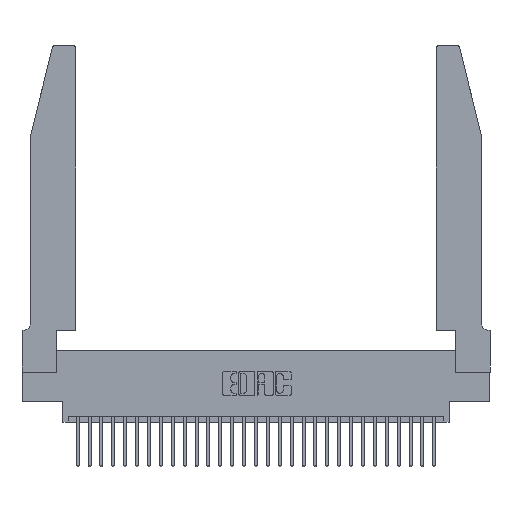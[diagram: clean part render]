
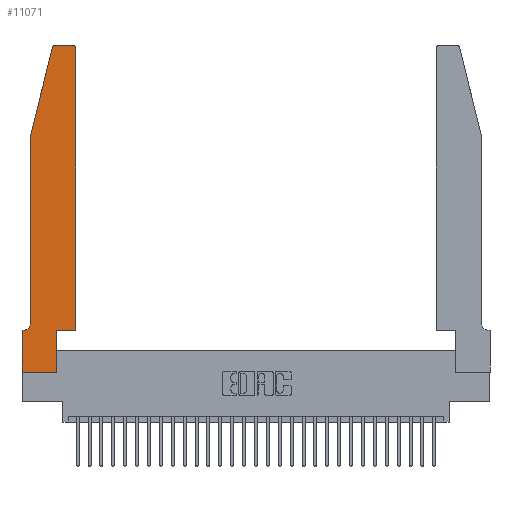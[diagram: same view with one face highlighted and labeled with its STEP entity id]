
A CAD part, top view. The second image highlights one B-rep face of the part: STEP entity #11071.
In plain terms, the highlighted planar face has unit normal (0, 0, 1).
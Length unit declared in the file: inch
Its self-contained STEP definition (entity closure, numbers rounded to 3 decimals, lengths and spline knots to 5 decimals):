
#51 = VECTOR ( 'NONE', #8601, 39.37008 ) ;
#865 = CARTESIAN_POINT ( 'NONE',  ( 0.0755, 2., 0.37 ) ) ;
#918 = LINE ( 'NONE', #25785, #24794 ) ;
#925 = LINE ( 'NONE', #14193, #5953 ) ;
#1254 = VERTEX_POINT ( 'NONE', #4482 ) ;
#1478 = ORIENTED_EDGE ( 'NONE', *, *, #30125, .T. ) ;
#1538 = DIRECTION ( 'NONE',  ( -1., 0., 0. ) ) ;
#1739 = CARTESIAN_POINT ( 'NONE',  ( 0.25487, 2.72718, 0.37 ) ) ;
#1925 = CARTESIAN_POINT ( 'NONE',  ( 0.0755, 0.42, 0.37 ) ) ;
#2300 = DIRECTION ( 'NONE',  ( 1., 0., 0. ) ) ;
#2882 = EDGE_CURVE ( 'NONE', #4517, #6202, #20335, .T. ) ;
#3135 = DIRECTION ( 'NONE',  ( -0.239, -0.971, 0. ) ) ;
#4482 = CARTESIAN_POINT ( 'NONE',  ( 0.0055, 0.35, 0.37 ) ) ;
#4517 = VERTEX_POINT ( 'NONE', #14096 ) ;
#4570 = DIRECTION ( 'NONE',  ( 0., 1., 0. ) ) ;
#5003 = LINE ( 'NONE', #26126, #16939 ) ;
#5183 = VECTOR ( 'NONE', #3135, 39.37008 ) ;
#5503 = VECTOR ( 'NONE', #7867, 39.37008 ) ;
#5849 = CARTESIAN_POINT ( 'NONE',  ( 0.2865, 0.35, 0.37 ) ) ;
#5953 = VECTOR ( 'NONE', #23533, 39.37008 ) ;
#6163 = ORIENTED_EDGE ( 'NONE', *, *, #2882, .T. ) ;
#6202 = VERTEX_POINT ( 'NONE', #11108 ) ;
#6253 = PLANE ( 'NONE',  #24596 ) ;
#6389 = EDGE_CURVE ( 'NONE', #26405, #24461, #918, .T. ) ;
#6524 = AXIS2_PLACEMENT_3D ( 'NONE', #22715, #8539, #25035 ) ;
#6534 = ORIENTED_EDGE ( 'NONE', *, *, #22010, .T. ) ;
#6748 = VECTOR ( 'NONE', #19270, 39.37008 ) ;
#7050 = VERTEX_POINT ( 'NONE', #28063 ) ;
#7363 = CIRCLE ( 'NONE', #26044, 0.07 ) ;
#7867 = DIRECTION ( 'NONE',  ( 0., -1., 0. ) ) ;
#8454 = CARTESIAN_POINT ( 'NONE',  ( 0., 0.35, 0.37 ) ) ;
#8539 = DIRECTION ( 'NONE',  ( 0., 0., 1. ) ) ;
#8601 = DIRECTION ( 'NONE',  ( -1., 0., 0. ) ) ;
#8653 = CARTESIAN_POINT ( 'NONE',  ( 0., 0.35, 0.37 ) ) ;
#8923 = ORIENTED_EDGE ( 'NONE', *, *, #17089, .T. ) ;
#9465 = CARTESIAN_POINT ( 'NONE',  ( 0.2865, 0., 0.37 ) ) ;
#10026 = LINE ( 'NONE', #17082, #21863 ) ;
#10037 = ORIENTED_EDGE ( 'NONE', *, *, #29590, .T. ) ;
#11040 = CARTESIAN_POINT ( 'NONE',  ( 0.4505, 2.72, 0.37 ) ) ;
#11071 = ADVANCED_FACE ( 'NONE', ( #20938 ), #6253, .T. ) ;
#11074 = DIRECTION ( 'NONE',  ( 1., 0., 0. ) ) ;
#11108 = CARTESIAN_POINT ( 'NONE',  ( 0.284, 2.75, 0.37 ) ) ;
#11179 = VERTEX_POINT ( 'NONE', #1739 ) ;
#11269 = ORIENTED_EDGE ( 'NONE', *, *, #19272, .T. ) ;
#12308 = ORIENTED_EDGE ( 'NONE', *, *, #18282, .T. ) ;
#12331 = ORIENTED_EDGE ( 'NONE', *, *, #25959, .T. ) ;
#12494 = ORIENTED_EDGE ( 'NONE', *, *, #13613, .T. ) ;
#12813 = VERTEX_POINT ( 'NONE', #865 ) ;
#13613 = EDGE_CURVE ( 'NONE', #11179, #12813, #28750, .T. ) ;
#14096 = CARTESIAN_POINT ( 'NONE',  ( 0.4205, 2.75, 0.37 ) ) ;
#14193 = CARTESIAN_POINT ( 'NONE',  ( 0.0755, 2., 0.37 ) ) ;
#14280 = EDGE_CURVE ( 'NONE', #25357, #7050, #18172, .T. ) ;
#14399 = LINE ( 'NONE', #18611, #26120 ) ;
#14452 = DIRECTION ( 'NONE',  ( 0., 1., 0. ) ) ;
#14781 = EDGE_CURVE ( 'NONE', #1254, #25357, #10026, .T. ) ;
#15969 = DIRECTION ( 'NONE',  ( 0., 0., -1. ) ) ;
#16662 = DIRECTION ( 'NONE',  ( 0., 0., 1. ) ) ;
#16939 = VECTOR ( 'NONE', #14452, 39.37008 ) ;
#16968 = VERTEX_POINT ( 'NONE', #1925 ) ;
#17082 = CARTESIAN_POINT ( 'NONE',  ( 0.0755, 0.35, 0.37 ) ) ;
#17089 = EDGE_CURVE ( 'NONE', #29001, #19119, #5003, .T. ) ;
#17452 = ORIENTED_EDGE ( 'NONE', *, *, #6389, .T. ) ;
#17460 = CARTESIAN_POINT ( 'NONE',  ( 0.0755, 2., 0.37 ) ) ;
#18172 = LINE ( 'NONE', #24375, #5503 ) ;
#18282 = EDGE_CURVE ( 'NONE', #24461, #4517, #21510, .T. ) ;
#18611 = CARTESIAN_POINT ( 'NONE',  ( 0., 0., 0.37 ) ) ;
#19119 = VERTEX_POINT ( 'NONE', #5849 ) ;
#19270 = DIRECTION ( 'NONE',  ( 1., 0., 0. ) ) ;
#19272 = EDGE_CURVE ( 'NONE', #16968, #1254, #7363, .T. ) ;
#19443 = DIRECTION ( 'NONE',  ( -1., 0., 0. ) ) ;
#20335 = LINE ( 'NONE', #22765, #51 ) ;
#20938 = FACE_OUTER_BOUND ( 'NONE', #28642, .T. ) ;
#20985 = DIRECTION ( 'NONE',  ( 1., 0., 0. ) ) ;
#21510 = CIRCLE ( 'NONE', #27764, 0.03 ) ;
#21863 = VECTOR ( 'NONE', #19443, 39.37008 ) ;
#22010 = EDGE_CURVE ( 'NONE', #6202, #11179, #28160, .T. ) ;
#22477 = CARTESIAN_POINT ( 'NONE',  ( 0.4505, 0.35, 0.37 ) ) ;
#22715 = CARTESIAN_POINT ( 'NONE',  ( 0.284, 2.72, 0.37 ) ) ;
#22765 = CARTESIAN_POINT ( 'NONE',  ( 0.2605, 2.75, 0.37 ) ) ;
#23533 = DIRECTION ( 'NONE',  ( 0., -1., 0. ) ) ;
#24375 = CARTESIAN_POINT ( 'NONE',  ( 0., 0., 0.37 ) ) ;
#24461 = VERTEX_POINT ( 'NONE', #11040 ) ;
#24596 = AXIS2_PLACEMENT_3D ( 'NONE', #8653, #25145, #11074 ) ;
#24794 = VECTOR ( 'NONE', #4570, 39.37008 ) ;
#25035 = DIRECTION ( 'NONE',  ( 1., 0., 0. ) ) ;
#25145 = DIRECTION ( 'NONE',  ( 0., 0., 1. ) ) ;
#25357 = VERTEX_POINT ( 'NONE', #8454 ) ;
#25561 = LINE ( 'NONE', #28512, #6748 ) ;
#25785 = CARTESIAN_POINT ( 'NONE',  ( 0.4505, 0.35, 0.37 ) ) ;
#25959 = EDGE_CURVE ( 'NONE', #7050, #29001, #14399, .T. ) ;
#26044 = AXIS2_PLACEMENT_3D ( 'NONE', #29889, #15969, #1538 ) ;
#26120 = VECTOR ( 'NONE', #20985, 39.37008 ) ;
#26126 = CARTESIAN_POINT ( 'NONE',  ( 0.2865, 0.35, 0.37 ) ) ;
#26405 = VERTEX_POINT ( 'NONE', #22477 ) ;
#27764 = AXIS2_PLACEMENT_3D ( 'NONE', #30582, #16662, #2300 ) ;
#28063 = CARTESIAN_POINT ( 'NONE',  ( 0., 0., 0.37 ) ) ;
#28160 = CIRCLE ( 'NONE', #6524, 0.03 ) ;
#28512 = CARTESIAN_POINT ( 'NONE',  ( 0.4505, 0.35, 0.37 ) ) ;
#28642 = EDGE_LOOP ( 'NONE', ( #6163, #6534, #12494, #1478, #11269, #29513, #30597, #12331, #8923, #10037, #17452, #12308 ) ) ;
#28750 = LINE ( 'NONE', #17460, #5183 ) ;
#29001 = VERTEX_POINT ( 'NONE', #9465 ) ;
#29513 = ORIENTED_EDGE ( 'NONE', *, *, #14781, .T. ) ;
#29590 = EDGE_CURVE ( 'NONE', #19119, #26405, #25561, .T. ) ;
#29889 = CARTESIAN_POINT ( 'NONE',  ( 0.0055, 0.42, 0.37 ) ) ;
#30125 = EDGE_CURVE ( 'NONE', #12813, #16968, #925, .T. ) ;
#30582 = CARTESIAN_POINT ( 'NONE',  ( 0.4205, 2.72, 0.37 ) ) ;
#30597 = ORIENTED_EDGE ( 'NONE', *, *, #14280, .T. ) ;
